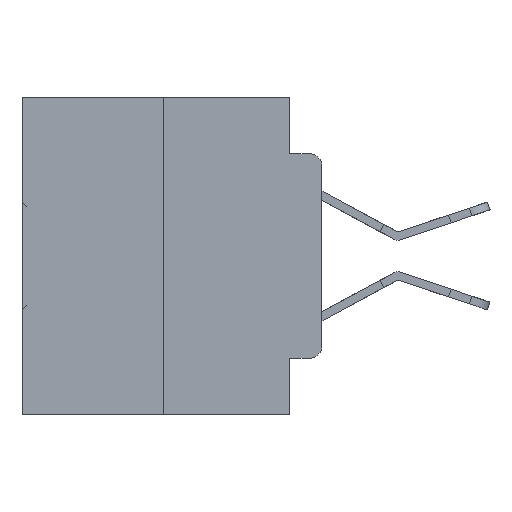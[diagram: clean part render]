
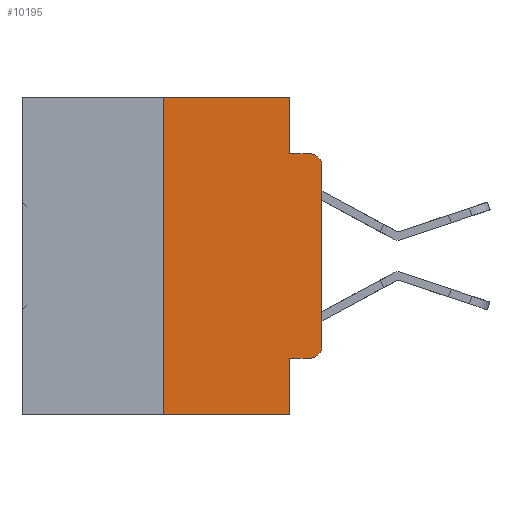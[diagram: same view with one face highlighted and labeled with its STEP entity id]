
A CAD part, left-side view. The second image highlights one B-rep face of the part: STEP entity #10195.
In plain terms, the highlighted planar face has unit normal (-1, 0, 0).
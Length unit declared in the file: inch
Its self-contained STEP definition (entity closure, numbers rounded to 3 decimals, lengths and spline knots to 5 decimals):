
#655 = LINE ( 'NONE', #11579, #14505 ) ;
#908 = DIRECTION ( 'NONE',  ( 0., 0., -1. ) ) ;
#1765 = DIRECTION ( 'NONE',  ( 0., -1., 0. ) ) ;
#1905 = ORIENTED_EDGE ( 'NONE', *, *, #3553, .T. ) ;
#2075 = AXIS2_PLACEMENT_3D ( 'NONE', #33580, #20167, #31098 ) ;
#2639 = AXIS2_PLACEMENT_3D ( 'NONE', #5349, #23842, #5186 ) ;
#2682 = VECTOR ( 'NONE', #4936, 39.37008 ) ;
#2720 = VERTEX_POINT ( 'NONE', #18692 ) ;
#3054 = DIRECTION ( 'NONE',  ( 0., -1., 0. ) ) ;
#3201 = LINE ( 'NONE', #3546, #16747 ) ;
#3419 = VECTOR ( 'NONE', #3054, 39.37008 ) ;
#3439 = ORIENTED_EDGE ( 'NONE', *, *, #34440, .F. ) ;
#3546 = CARTESIAN_POINT ( 'NONE',  ( 0., 0.051, 0. ) ) ;
#3553 = EDGE_CURVE ( 'NONE', #6254, #7402, #10810, .T. ) ;
#4218 = CARTESIAN_POINT ( 'NONE',  ( 0., 0., 0. ) ) ;
#4264 = VERTEX_POINT ( 'NONE', #10142 ) ;
#4271 = EDGE_CURVE ( 'NONE', #22531, #13349, #25471, .T. ) ;
#4672 = ORIENTED_EDGE ( 'NONE', *, *, #11627, .T. ) ;
#4741 = LINE ( 'NONE', #4218, #2682 ) ;
#4936 = DIRECTION ( 'NONE',  ( 0., 0., 1. ) ) ;
#5173 = VERTEX_POINT ( 'NONE', #29110 ) ;
#5186 = DIRECTION ( 'NONE',  ( 0., 0., -1. ) ) ;
#5349 = CARTESIAN_POINT ( 'NONE',  ( 0., 0.02, -0.3915 ) ) ;
#5398 = DIRECTION ( 'NONE',  ( 0., 0., 1. ) ) ;
#5824 = VERTEX_POINT ( 'NONE', #33749 ) ;
#6170 = VERTEX_POINT ( 'NONE', #16573 ) ;
#6254 = VERTEX_POINT ( 'NONE', #33186 ) ;
#6794 = CARTESIAN_POINT ( 'NONE',  ( 0., 0.02, -0.4115 ) ) ;
#6857 = ORIENTED_EDGE ( 'NONE', *, *, #22049, .F. ) ;
#7206 = VECTOR ( 'NONE', #27260, 39.37008 ) ;
#7338 = ORIENTED_EDGE ( 'NONE', *, *, #26227, .T. ) ;
#7402 = VERTEX_POINT ( 'NONE', #8847 ) ;
#8847 = CARTESIAN_POINT ( 'NONE',  ( 0., 0.051, -0.5 ) ) ;
#9870 = ORIENTED_EDGE ( 'NONE', *, *, #11350, .T. ) ;
#10142 = CARTESIAN_POINT ( 'NONE',  ( 0., 0.051, 0. ) ) ;
#10195 = ADVANCED_FACE ( 'NONE', ( #17513 ), #17348, .F. ) ;
#10646 = DIRECTION ( 'NONE',  ( 0., -1., 0. ) ) ;
#10798 = LINE ( 'NONE', #34305, #12081 ) ;
#10810 = LINE ( 'NONE', #27194, #3419 ) ;
#11050 = CARTESIAN_POINT ( 'NONE',  ( 0., 0.051, 0. ) ) ;
#11350 = EDGE_CURVE ( 'NONE', #5824, #22531, #4741, .T. ) ;
#11579 = CARTESIAN_POINT ( 'NONE',  ( 0., 0.051, -0.4115 ) ) ;
#11627 = EDGE_CURVE ( 'NONE', #5173, #30685, #655, .T. ) ;
#11735 = ORIENTED_EDGE ( 'NONE', *, *, #22480, .F. ) ;
#12081 = VECTOR ( 'NONE', #10646, 39.37008 ) ;
#12862 = CARTESIAN_POINT ( 'NONE',  ( 0., 0.473, 0. ) ) ;
#12979 = CARTESIAN_POINT ( 'NONE',  ( 0., 0.25, 0. ) ) ;
#13349 = VERTEX_POINT ( 'NONE', #32071 ) ;
#14131 = CARTESIAN_POINT ( 'NONE',  ( 0., 0., -0.1085 ) ) ;
#14505 = VECTOR ( 'NONE', #33277, 39.37008 ) ;
#16573 = CARTESIAN_POINT ( 'NONE',  ( 0., 0.051, -0.0885 ) ) ;
#16747 = VECTOR ( 'NONE', #908, 39.37008 ) ;
#17308 = ORIENTED_EDGE ( 'NONE', *, *, #27306, .F. ) ;
#17348 = PLANE ( 'NONE',  #2075 ) ;
#17513 = FACE_OUTER_BOUND ( 'NONE', #18420, .T. ) ;
#17584 = AXIS2_PLACEMENT_3D ( 'NONE', #34318, #31644, #34481 ) ;
#18420 = EDGE_LOOP ( 'NONE', ( #9870, #24540, #11735, #26321, #3439, #6857, #1905, #17308, #4672, #7338 ) ) ;
#18692 = CARTESIAN_POINT ( 'NONE',  ( 0., 0.25, 0. ) ) ;
#19275 = EDGE_CURVE ( 'NONE', #4264, #6170, #3201, .T. ) ;
#20167 = DIRECTION ( 'NONE',  ( 1., 0., 0. ) ) ;
#22049 = EDGE_CURVE ( 'NONE', #6254, #2720, #24237, .T. ) ;
#22463 = LINE ( 'NONE', #11050, #7206 ) ;
#22480 = EDGE_CURVE ( 'NONE', #6170, #13349, #10798, .T. ) ;
#22531 = VERTEX_POINT ( 'NONE', #14131 ) ;
#23842 = DIRECTION ( 'NONE',  ( -1., 0., 0. ) ) ;
#23859 = VECTOR ( 'NONE', #5398, 39.37008 ) ;
#24237 = LINE ( 'NONE', #12979, #23859 ) ;
#24540 = ORIENTED_EDGE ( 'NONE', *, *, #4271, .T. ) ;
#24576 = CIRCLE ( 'NONE', #2639, 0.02 ) ;
#25471 = CIRCLE ( 'NONE', #17584, 0.02 ) ;
#26227 = EDGE_CURVE ( 'NONE', #30685, #5824, #24576, .T. ) ;
#26321 = ORIENTED_EDGE ( 'NONE', *, *, #19275, .F. ) ;
#27194 = CARTESIAN_POINT ( 'NONE',  ( 0., 0.473, -0.5 ) ) ;
#27260 = DIRECTION ( 'NONE',  ( 0., 0., -1. ) ) ;
#27306 = EDGE_CURVE ( 'NONE', #5173, #7402, #22463, .T. ) ;
#28575 = LINE ( 'NONE', #12862, #34135 ) ;
#29110 = CARTESIAN_POINT ( 'NONE',  ( 0., 0.051, -0.4115 ) ) ;
#30685 = VERTEX_POINT ( 'NONE', #6794 ) ;
#31098 = DIRECTION ( 'NONE',  ( 0., 0., -1. ) ) ;
#31644 = DIRECTION ( 'NONE',  ( -1., 0., 0. ) ) ;
#32071 = CARTESIAN_POINT ( 'NONE',  ( 0., 0.02, -0.0885 ) ) ;
#33186 = CARTESIAN_POINT ( 'NONE',  ( 0., 0.25, -0.5 ) ) ;
#33277 = DIRECTION ( 'NONE',  ( 0., -1., 0. ) ) ;
#33580 = CARTESIAN_POINT ( 'NONE',  ( 0., 0.473, 0. ) ) ;
#33749 = CARTESIAN_POINT ( 'NONE',  ( 0., 0., -0.3915 ) ) ;
#34135 = VECTOR ( 'NONE', #1765, 39.37008 ) ;
#34305 = CARTESIAN_POINT ( 'NONE',  ( 0., 0.051, -0.0885 ) ) ;
#34318 = CARTESIAN_POINT ( 'NONE',  ( 0., 0.02, -0.1085 ) ) ;
#34440 = EDGE_CURVE ( 'NONE', #2720, #4264, #28575, .T. ) ;
#34481 = DIRECTION ( 'NONE',  ( 0., 0., -1. ) ) ;
